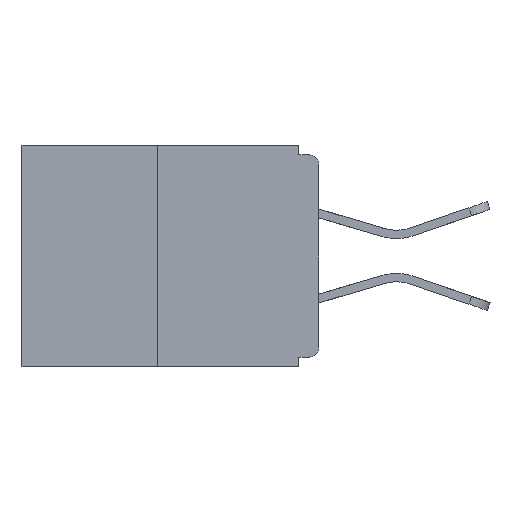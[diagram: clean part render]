
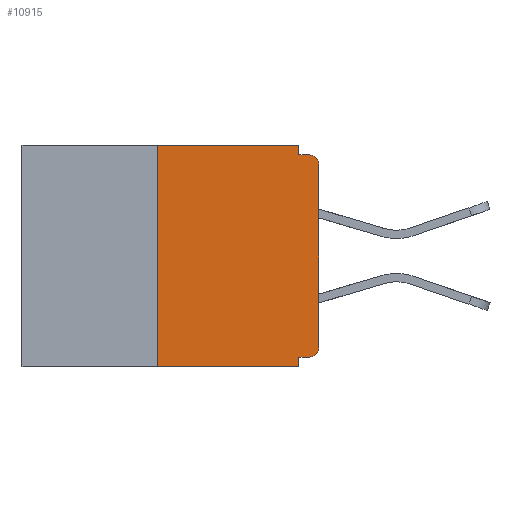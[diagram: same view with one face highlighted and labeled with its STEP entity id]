
A CAD part, left-side view. The second image highlights one B-rep face of the part: STEP entity #10915.
In plain terms, the highlighted planar face has unit normal (-1, 0, 0).
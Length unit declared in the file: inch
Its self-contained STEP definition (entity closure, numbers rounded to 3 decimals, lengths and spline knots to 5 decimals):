
#154 = PLANE ( 'NONE',  #14998 ) ;
#178 = CARTESIAN_POINT ( 'NONE',  ( 0., 0.25, -0.343 ) ) ;
#182 = ORIENTED_EDGE ( 'NONE', *, *, #5824, .T. ) ;
#753 = CARTESIAN_POINT ( 'NONE',  ( 0., 0., -0.313 ) ) ;
#1230 = CARTESIAN_POINT ( 'NONE',  ( 0., 0.015, -0.03 ) ) ;
#1420 = ORIENTED_EDGE ( 'NONE', *, *, #3576, .T. ) ;
#1552 = DIRECTION ( 'NONE',  ( 0., 0., -1. ) ) ;
#1753 = DIRECTION ( 'NONE',  ( 0., -1., 0. ) ) ;
#2004 = LINE ( 'NONE', #7688, #13433 ) ;
#2394 = EDGE_CURVE ( 'NONE', #16997, #9506, #13526, .T. ) ;
#2589 = EDGE_CURVE ( 'NONE', #3793, #14201, #14030, .T. ) ;
#3160 = DIRECTION ( 'NONE',  ( 0., 0., 1. ) ) ;
#3365 = DIRECTION ( 'NONE',  ( 0., 0., 1. ) ) ;
#3366 = CARTESIAN_POINT ( 'NONE',  ( 0., 0., -0.015 ) ) ;
#3458 = DIRECTION ( 'NONE',  ( 0., -1., 0. ) ) ;
#3576 = EDGE_CURVE ( 'NONE', #9506, #6949, #11332, .T. ) ;
#3793 = VERTEX_POINT ( 'NONE', #17080 ) ;
#4291 = FACE_OUTER_BOUND ( 'NONE', #16518, .T. ) ;
#4431 = ORIENTED_EDGE ( 'NONE', *, *, #2394, .T. ) ;
#4493 = DIRECTION ( 'NONE',  ( -1., 0., 0. ) ) ;
#4813 = DIRECTION ( 'NONE',  ( 0., 1., 0. ) ) ;
#5824 = EDGE_CURVE ( 'NONE', #10531, #14201, #17350, .T. ) ;
#6028 = VERTEX_POINT ( 'NONE', #9424 ) ;
#6513 = DIRECTION ( 'NONE',  ( 0., 0., -1. ) ) ;
#6918 = EDGE_CURVE ( 'NONE', #6028, #9135, #16180, .T. ) ;
#6949 = VERTEX_POINT ( 'NONE', #20197 ) ;
#7404 = CARTESIAN_POINT ( 'NONE',  ( 0., 0.015, -0.328 ) ) ;
#7540 = DIRECTION ( 'NONE',  ( 0., -1., 0. ) ) ;
#7688 = CARTESIAN_POINT ( 'NONE',  ( 0., 0.46, 0. ) ) ;
#7742 = VECTOR ( 'NONE', #4813, 39.37008 ) ;
#8248 = VECTOR ( 'NONE', #6513, 39.37008 ) ;
#8799 = CARTESIAN_POINT ( 'NONE',  ( 0., 0.25, 0. ) ) ;
#8823 = CARTESIAN_POINT ( 'NONE',  ( 0., 0.46, 0. ) ) ;
#9059 = EDGE_CURVE ( 'NONE', #11596, #6028, #2004, .T. ) ;
#9135 = VERTEX_POINT ( 'NONE', #21872 ) ;
#9149 = CIRCLE ( 'NONE', #19162, 0.015 ) ;
#9214 = CARTESIAN_POINT ( 'NONE',  ( 0., 0.015, -0.313 ) ) ;
#9424 = CARTESIAN_POINT ( 'NONE',  ( 0., 0.031, 0. ) ) ;
#9506 = VERTEX_POINT ( 'NONE', #13201 ) ;
#9581 = EDGE_CURVE ( 'NONE', #9135, #6949, #14197, .T. ) ;
#9756 = CARTESIAN_POINT ( 'NONE',  ( 0., 0.25, 0. ) ) ;
#10531 = VERTEX_POINT ( 'NONE', #178 ) ;
#10915 = ADVANCED_FACE ( 'NONE', ( #4291 ), #154, .F. ) ;
#11041 = EDGE_CURVE ( 'NONE', #16322, #16997, #9149, .T. ) ;
#11332 = CIRCLE ( 'NONE', #21792, 0.015 ) ;
#11570 = ORIENTED_EDGE ( 'NONE', *, *, #11041, .T. ) ;
#11596 = VERTEX_POINT ( 'NONE', #8799 ) ;
#11899 = CARTESIAN_POINT ( 'NONE',  ( 0., 0.46, -0.343 ) ) ;
#12174 = DIRECTION ( 'NONE',  ( 0., 0., -1. ) ) ;
#12187 = CARTESIAN_POINT ( 'NONE',  ( 0., 0., 0. ) ) ;
#12323 = EDGE_CURVE ( 'NONE', #16322, #3793, #13314, .T. ) ;
#12602 = VECTOR ( 'NONE', #1753, 39.37008 ) ;
#12787 = VECTOR ( 'NONE', #3458, 39.37008 ) ;
#13146 = CARTESIAN_POINT ( 'NONE',  ( 0., 0.031, -0.343 ) ) ;
#13201 = CARTESIAN_POINT ( 'NONE',  ( 0., 0., -0.03 ) ) ;
#13314 = LINE ( 'NONE', #14850, #7742 ) ;
#13316 = LINE ( 'NONE', #9756, #21888 ) ;
#13433 = VECTOR ( 'NONE', #7540, 39.37008 ) ;
#13526 = LINE ( 'NONE', #12187, #17508 ) ;
#14030 = LINE ( 'NONE', #21799, #8248 ) ;
#14197 = LINE ( 'NONE', #3366, #12602 ) ;
#14201 = VERTEX_POINT ( 'NONE', #13146 ) ;
#14850 = CARTESIAN_POINT ( 'NONE',  ( 0., 0., -0.328 ) ) ;
#14998 = AXIS2_PLACEMENT_3D ( 'NONE', #8823, #20711, #22054 ) ;
#15010 = ORIENTED_EDGE ( 'NONE', *, *, #9581, .F. ) ;
#15295 = DIRECTION ( 'NONE',  ( -1., 0., 0. ) ) ;
#15962 = ORIENTED_EDGE ( 'NONE', *, *, #6918, .F. ) ;
#16180 = LINE ( 'NONE', #20050, #20503 ) ;
#16322 = VERTEX_POINT ( 'NONE', #7404 ) ;
#16470 = DIRECTION ( 'NONE',  ( 0., 0., -1. ) ) ;
#16518 = EDGE_LOOP ( 'NONE', ( #21627, #18842, #182, #19472, #19664, #11570, #4431, #1420, #15010, #15962 ) ) ;
#16997 = VERTEX_POINT ( 'NONE', #753 ) ;
#17080 = CARTESIAN_POINT ( 'NONE',  ( 0., 0.031, -0.328 ) ) ;
#17350 = LINE ( 'NONE', #11899, #12787 ) ;
#17508 = VECTOR ( 'NONE', #3365, 39.37008 ) ;
#17772 = EDGE_CURVE ( 'NONE', #10531, #11596, #13316, .T. ) ;
#18842 = ORIENTED_EDGE ( 'NONE', *, *, #17772, .F. ) ;
#19162 = AXIS2_PLACEMENT_3D ( 'NONE', #9214, #15295, #12174 ) ;
#19472 = ORIENTED_EDGE ( 'NONE', *, *, #2589, .F. ) ;
#19664 = ORIENTED_EDGE ( 'NONE', *, *, #12323, .F. ) ;
#20050 = CARTESIAN_POINT ( 'NONE',  ( 0., 0.031, 0. ) ) ;
#20197 = CARTESIAN_POINT ( 'NONE',  ( 0., 0.015, -0.015 ) ) ;
#20503 = VECTOR ( 'NONE', #1552, 39.37008 ) ;
#20711 = DIRECTION ( 'NONE',  ( 1., 0., 0. ) ) ;
#21627 = ORIENTED_EDGE ( 'NONE', *, *, #9059, .F. ) ;
#21792 = AXIS2_PLACEMENT_3D ( 'NONE', #1230, #4493, #16470 ) ;
#21799 = CARTESIAN_POINT ( 'NONE',  ( 0., 0.031, -0.343 ) ) ;
#21872 = CARTESIAN_POINT ( 'NONE',  ( 0., 0.031, -0.015 ) ) ;
#21888 = VECTOR ( 'NONE', #3160, 39.37008 ) ;
#22054 = DIRECTION ( 'NONE',  ( 0., 0., -1. ) ) ;
